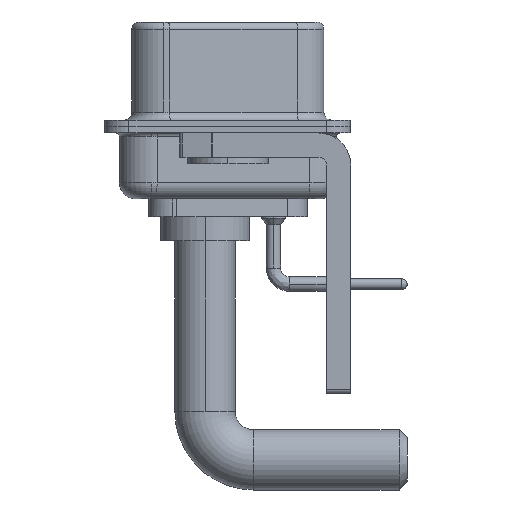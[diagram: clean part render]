
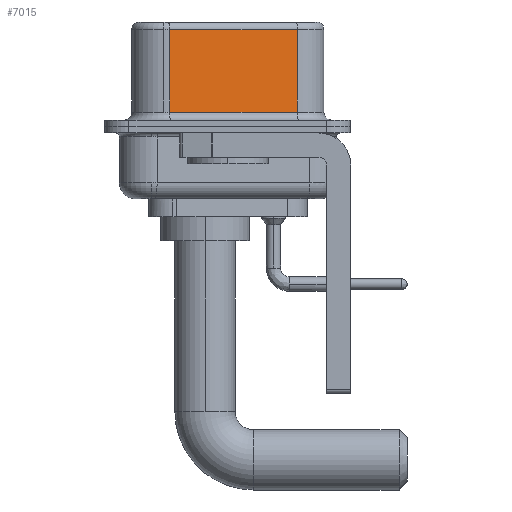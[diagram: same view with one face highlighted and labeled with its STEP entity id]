
A CAD part, left-side view. The second image highlights one B-rep face of the part: STEP entity #7015.
In plain terms, the highlighted planar face has unit normal (-0.985, -0.174, 0).
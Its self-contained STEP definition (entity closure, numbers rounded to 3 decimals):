
#234 = ORIENTED_EDGE ( 'NONE', *, *, #10539, .T. ) ;
#1123 = DIRECTION ( 'NONE',  ( -0.174, 0.985, 0. ) ) ;
#2849 = VECTOR ( 'NONE', #5363, 1000. ) ;
#3053 = EDGE_CURVE ( 'NONE', #15171, #14496, #10641, .T. ) ;
#3127 = CARTESIAN_POINT ( 'NONE',  ( 3.73, 3.628, 6.52 ) ) ;
#5143 = EDGE_CURVE ( 'NONE', #15171, #20579, #7482, .T. ) ;
#5363 = DIRECTION ( 'NONE',  ( 0., 0., -1. ) ) ;
#5952 = PLANE ( 'NONE',  #17319 ) ;
#7015 = ADVANCED_FACE ( 'NONE', ( #14031 ), #5952, .F. ) ;
#7092 = CARTESIAN_POINT ( 'NONE',  ( 3.73, 3.628, 0.9 ) ) ;
#7168 = ORIENTED_EDGE ( 'NONE', *, *, #8087, .T. ) ;
#7482 = LINE ( 'NONE', #11233, #2849 ) ;
#7815 = ORIENTED_EDGE ( 'NONE', *, *, #3053, .T. ) ;
#8087 = EDGE_CURVE ( 'NONE', #14496, #20050, #12598, .T. ) ;
#8938 = CARTESIAN_POINT ( 'NONE',  ( 5.132, -4.322, 0.9 ) ) ;
#9710 = VECTOR ( 'NONE', #1123, 1000. ) ;
#10539 = EDGE_CURVE ( 'NONE', #20050, #20579, #21500, .T. ) ;
#10641 = LINE ( 'NONE', #14229, #9710 ) ;
#10848 = CARTESIAN_POINT ( 'NONE',  ( 5.132, -4.322, 6.02 ) ) ;
#11233 = CARTESIAN_POINT ( 'NONE',  ( 5.132, -4.322, 6.52 ) ) ;
#12041 = DIRECTION ( 'NONE',  ( 0.985, 0.174, 0. ) ) ;
#12463 = ORIENTED_EDGE ( 'NONE', *, *, #5143, .F. ) ;
#12593 = VECTOR ( 'NONE', #21687, 1000. ) ;
#12598 = LINE ( 'NONE', #3127, #12593 ) ;
#14031 = FACE_OUTER_BOUND ( 'NONE', #15272, .T. ) ;
#14229 = CARTESIAN_POINT ( 'NONE',  ( 5.132, -4.322, 6.02 ) ) ;
#14496 = VERTEX_POINT ( 'NONE', #23071 ) ;
#15171 = VERTEX_POINT ( 'NONE', #10848 ) ;
#15272 = EDGE_LOOP ( 'NONE', ( #12463, #7815, #7168, #234 ) ) ;
#17017 = VECTOR ( 'NONE', #24111, 1000. ) ;
#17319 = AXIS2_PLACEMENT_3D ( 'NONE', #21137, #12041, #21624 ) ;
#17706 = CARTESIAN_POINT ( 'NONE',  ( 5.132, -4.322, 0.9 ) ) ;
#20050 = VERTEX_POINT ( 'NONE', #7092 ) ;
#20579 = VERTEX_POINT ( 'NONE', #17706 ) ;
#21137 = CARTESIAN_POINT ( 'NONE',  ( 5.132, -4.322, 6.52 ) ) ;
#21500 = LINE ( 'NONE', #8938, #17017 ) ;
#21624 = DIRECTION ( 'NONE',  ( -0.174, 0.985, 0. ) ) ;
#21687 = DIRECTION ( 'NONE',  ( 0., 0., -1. ) ) ;
#23071 = CARTESIAN_POINT ( 'NONE',  ( 3.73, 3.628, 6.02 ) ) ;
#24111 = DIRECTION ( 'NONE',  ( 0.174, -0.985, 0. ) ) ;
